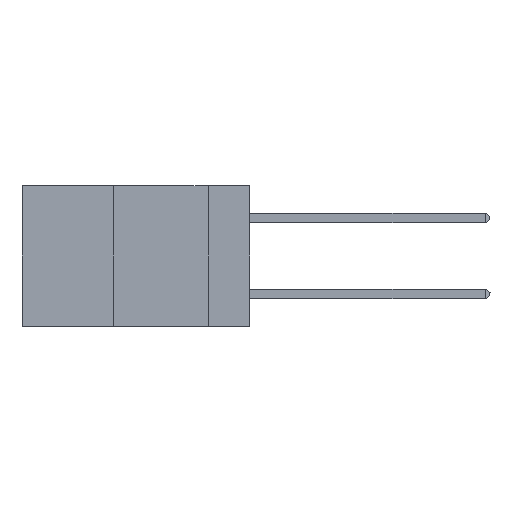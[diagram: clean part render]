
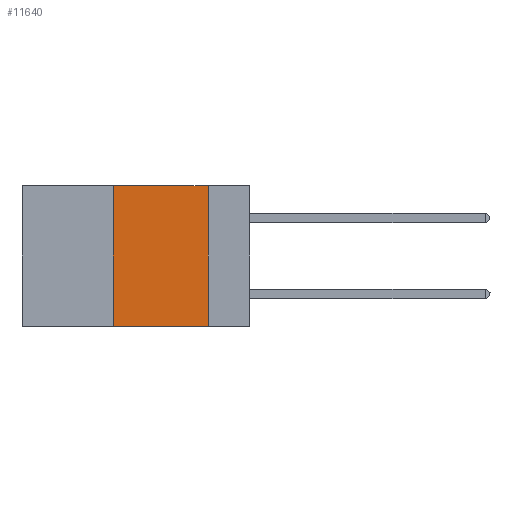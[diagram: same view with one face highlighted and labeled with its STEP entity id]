
A CAD part, left-side view. The second image highlights one B-rep face of the part: STEP entity #11640.
In plain terms, the highlighted planar face has unit normal (-1, 0, 0).
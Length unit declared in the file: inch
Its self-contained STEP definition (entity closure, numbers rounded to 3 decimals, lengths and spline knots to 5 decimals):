
#170 = CARTESIAN_POINT ( 'NONE',  ( 0., 0.11, 0. ) ) ;
#173 = CARTESIAN_POINT ( 'NONE',  ( 0., 0.11, 0. ) ) ;
#895 = ORIENTED_EDGE ( 'NONE', *, *, #1422, .F. ) ;
#1422 = EDGE_CURVE ( 'NONE', #8743, #19440, #19467, .T. ) ;
#1702 = VERTEX_POINT ( 'NONE', #8953 ) ;
#1736 = AXIS2_PLACEMENT_3D ( 'NONE', #18470, #13216, #11596 ) ;
#3270 = DIRECTION ( 'NONE',  ( 0., -1., 0. ) ) ;
#5158 = VECTOR ( 'NONE', #18778, 39.37008 ) ;
#7818 = CARTESIAN_POINT ( 'NONE',  ( 0., 0.36, 0. ) ) ;
#8149 = CARTESIAN_POINT ( 'NONE',  ( 0., 0.6, 0. ) ) ;
#8530 = CARTESIAN_POINT ( 'NONE',  ( 0., 0.36, 0. ) ) ;
#8743 = VERTEX_POINT ( 'NONE', #8530 ) ;
#8953 = CARTESIAN_POINT ( 'NONE',  ( 0., 0.11, -0.37 ) ) ;
#11019 = VERTEX_POINT ( 'NONE', #18839 ) ;
#11421 = LINE ( 'NONE', #22596, #15588 ) ;
#11596 = DIRECTION ( 'NONE',  ( 0., 0., -1. ) ) ;
#11640 = ADVANCED_FACE ( 'NONE', ( #21087 ), #20360, .F. ) ;
#13216 = DIRECTION ( 'NONE',  ( 1., 0., 0. ) ) ;
#13222 = LINE ( 'NONE', #7818, #19026 ) ;
#14888 = EDGE_CURVE ( 'NONE', #11019, #8743, #13222, .T. ) ;
#15052 = LINE ( 'NONE', #173, #21886 ) ;
#15143 = ORIENTED_EDGE ( 'NONE', *, *, #21885, .T. ) ;
#15588 = VECTOR ( 'NONE', #3270, 39.37008 ) ;
#16667 = DIRECTION ( 'NONE',  ( 0., 0., 1. ) ) ;
#17092 = ORIENTED_EDGE ( 'NONE', *, *, #18317, .F. ) ;
#18017 = DIRECTION ( 'NONE',  ( 0., 0., -1. ) ) ;
#18317 = EDGE_CURVE ( 'NONE', #19440, #1702, #15052, .T. ) ;
#18470 = CARTESIAN_POINT ( 'NONE',  ( 0., 0.6, 0. ) ) ;
#18778 = DIRECTION ( 'NONE',  ( 0., -1., 0. ) ) ;
#18839 = CARTESIAN_POINT ( 'NONE',  ( 0., 0.36, -0.37 ) ) ;
#19026 = VECTOR ( 'NONE', #16667, 39.37008 ) ;
#19440 = VERTEX_POINT ( 'NONE', #170 ) ;
#19467 = LINE ( 'NONE', #8149, #5158 ) ;
#19933 = EDGE_LOOP ( 'NONE', ( #17092, #895, #20747, #15143 ) ) ;
#20360 = PLANE ( 'NONE',  #1736 ) ;
#20747 = ORIENTED_EDGE ( 'NONE', *, *, #14888, .F. ) ;
#21087 = FACE_OUTER_BOUND ( 'NONE', #19933, .T. ) ;
#21885 = EDGE_CURVE ( 'NONE', #11019, #1702, #11421, .T. ) ;
#21886 = VECTOR ( 'NONE', #18017, 39.37008 ) ;
#22596 = CARTESIAN_POINT ( 'NONE',  ( 0., 0.6, -0.37 ) ) ;
